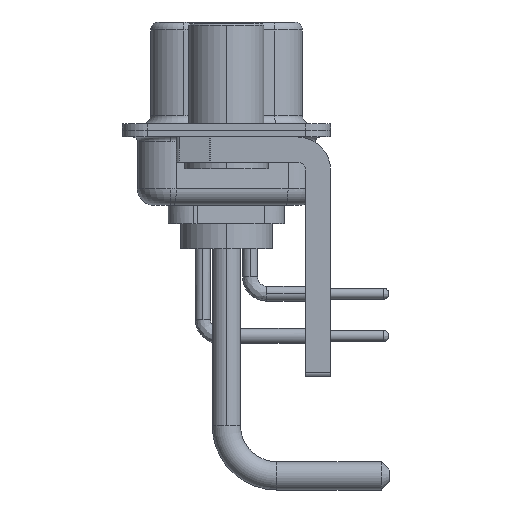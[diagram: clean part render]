
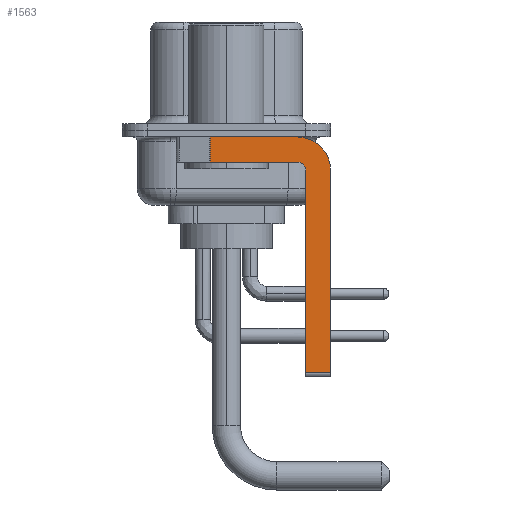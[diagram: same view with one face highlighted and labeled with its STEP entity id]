
A CAD part, left-side view. The second image highlights one B-rep face of the part: STEP entity #1563.
In plain terms, the highlighted planar face has unit normal (-1, 0, 0).
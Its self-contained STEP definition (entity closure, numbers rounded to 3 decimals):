
#76 = VERTEX_POINT ( 'NONE', #13917 ) ;
#178 = ORIENTED_EDGE ( 'NONE', *, *, #5137, .F. ) ;
#383 = DIRECTION ( 'NONE',  ( 0., 0., -1. ) ) ;
#1247 = CARTESIAN_POINT ( 'NONE',  ( -2.9, -6.25, -14.55 ) ) ;
#1453 = CARTESIAN_POINT ( 'NONE',  ( -2.9, -4.25, -14.55 ) ) ;
#1563 = ADVANCED_FACE ( 'NONE', ( #12649 ), #16523, .F. ) ;
#1885 = CARTESIAN_POINT ( 'NONE',  ( -2.9, -4.75, -14.8 ) ) ;
#3300 = ORIENTED_EDGE ( 'NONE', *, *, #23080, .F. ) ;
#3477 = AXIS2_PLACEMENT_3D ( 'NONE', #25223, #18991, #8528 ) ;
#3859 = ORIENTED_EDGE ( 'NONE', *, *, #17065, .F. ) ;
#4172 = VECTOR ( 'NONE', #16879, 1000. ) ;
#5053 = AXIS2_PLACEMENT_3D ( 'NONE', #16094, #15956, #24111 ) ;
#5137 = EDGE_CURVE ( 'NONE', #76, #15949, #5577, .T. ) ;
#5577 = LINE ( 'NONE', #7764, #16420 ) ;
#5732 = CARTESIAN_POINT ( 'NONE',  ( -2.9, -4.25, -1.9 ) ) ;
#5741 = EDGE_CURVE ( 'NONE', #16146, #15180, #10727, .T. ) ;
#6554 = DIRECTION ( 'NONE',  ( 1., 0., 0. ) ) ;
#6613 = DIRECTION ( 'NONE',  ( 0., -1., 0. ) ) ;
#6763 = VECTOR ( 'NONE', #9571, 1000. ) ;
#7390 = CARTESIAN_POINT ( 'NONE',  ( -2.9, 0.978, -1.9 ) ) ;
#7634 = DIRECTION ( 'NONE',  ( 0., 0., -1. ) ) ;
#7649 = EDGE_CURVE ( 'NONE', #26521, #23446, #16925, .T. ) ;
#7764 = CARTESIAN_POINT ( 'NONE',  ( -2.9, -6.25, -2.4 ) ) ;
#7875 = CIRCLE ( 'NONE', #11379, 2. ) ;
#8079 = VERTEX_POINT ( 'NONE', #24218 ) ;
#8134 = CARTESIAN_POINT ( 'NONE',  ( -2.9, 3., -0.4 ) ) ;
#8528 = DIRECTION ( 'NONE',  ( 0., 0., -1. ) ) ;
#9571 = DIRECTION ( 'NONE',  ( 0., -1., 0. ) ) ;
#10612 = ORIENTED_EDGE ( 'NONE', *, *, #27224, .T. ) ;
#10727 = LINE ( 'NONE', #8134, #20542 ) ;
#10857 = ORIENTED_EDGE ( 'NONE', *, *, #5741, .F. ) ;
#11213 = ORIENTED_EDGE ( 'NONE', *, *, #23512, .T. ) ;
#11379 = AXIS2_PLACEMENT_3D ( 'NONE', #23223, #6554, #14946 ) ;
#11519 = LINE ( 'NONE', #21604, #15710 ) ;
#12649 = FACE_OUTER_BOUND ( 'NONE', #21881, .T. ) ;
#12959 = EDGE_CURVE ( 'NONE', #15180, #76, #7875, .T. ) ;
#13601 = CARTESIAN_POINT ( 'NONE',  ( -2.9, -4.25, -0.4 ) ) ;
#13917 = CARTESIAN_POINT ( 'NONE',  ( -2.9, -6.25, -2.4 ) ) ;
#14946 = DIRECTION ( 'NONE',  ( 0., 0., -1. ) ) ;
#15180 = VERTEX_POINT ( 'NONE', #13601 ) ;
#15710 = VECTOR ( 'NONE', #383, 1000. ) ;
#15949 = VERTEX_POINT ( 'NONE', #1247 ) ;
#15956 = DIRECTION ( 'NONE',  ( -1., 0., 0. ) ) ;
#16094 = CARTESIAN_POINT ( 'NONE',  ( -2.9, -4.25, -2.4 ) ) ;
#16146 = VERTEX_POINT ( 'NONE', #22736 ) ;
#16176 = CARTESIAN_POINT ( 'NONE',  ( -2.9, -4.25, -1.9 ) ) ;
#16420 = VECTOR ( 'NONE', #7634, 1000. ) ;
#16523 = PLANE ( 'NONE',  #3477 ) ;
#16750 = LINE ( 'NONE', #1885, #4172 ) ;
#16879 = DIRECTION ( 'NONE',  ( 0., 0., 1. ) ) ;
#16925 = CIRCLE ( 'NONE', #5053, 0.5 ) ;
#17065 = EDGE_CURVE ( 'NONE', #23446, #17392, #25017, .T. ) ;
#17392 = VERTEX_POINT ( 'NONE', #7390 ) ;
#18542 = VECTOR ( 'NONE', #20317, 1000. ) ;
#18991 = DIRECTION ( 'NONE',  ( 1., 0., 0. ) ) ;
#19410 = ORIENTED_EDGE ( 'NONE', *, *, #7649, .F. ) ;
#20317 = DIRECTION ( 'NONE',  ( 0., 1., 0. ) ) ;
#20542 = VECTOR ( 'NONE', #6613, 1000. ) ;
#21604 = CARTESIAN_POINT ( 'NONE',  ( -2.9, 0.978, -1.9 ) ) ;
#21881 = EDGE_LOOP ( 'NONE', ( #10857, #10612, #3859, #19410, #3300, #11213, #178, #24327 ) ) ;
#22116 = LINE ( 'NONE', #1453, #6763 ) ;
#22736 = CARTESIAN_POINT ( 'NONE',  ( -2.9, 0.978, -0.4 ) ) ;
#22934 = CARTESIAN_POINT ( 'NONE',  ( -2.9, -4.75, -2.4 ) ) ;
#23080 = EDGE_CURVE ( 'NONE', #8079, #26521, #16750, .T. ) ;
#23223 = CARTESIAN_POINT ( 'NONE',  ( -2.9, -4.25, -2.4 ) ) ;
#23446 = VERTEX_POINT ( 'NONE', #5732 ) ;
#23512 = EDGE_CURVE ( 'NONE', #8079, #15949, #22116, .T. ) ;
#24111 = DIRECTION ( 'NONE',  ( 0., 0., 1. ) ) ;
#24218 = CARTESIAN_POINT ( 'NONE',  ( -2.9, -4.75, -14.55 ) ) ;
#24327 = ORIENTED_EDGE ( 'NONE', *, *, #12959, .F. ) ;
#25017 = LINE ( 'NONE', #16176, #18542 ) ;
#25223 = CARTESIAN_POINT ( 'NONE',  ( -2.9, -4.25, -2.4 ) ) ;
#26521 = VERTEX_POINT ( 'NONE', #22934 ) ;
#27224 = EDGE_CURVE ( 'NONE', #16146, #17392, #11519, .T. ) ;
